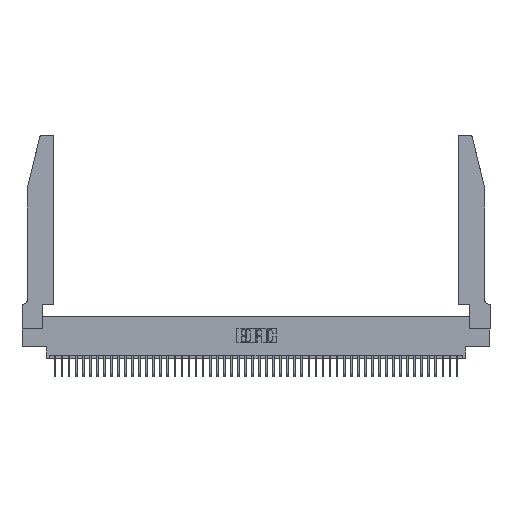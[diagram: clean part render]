
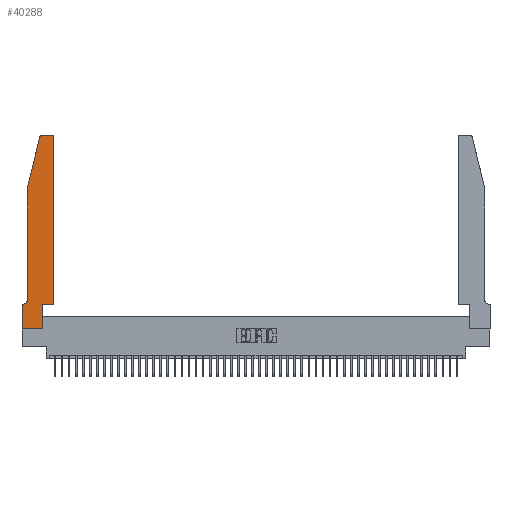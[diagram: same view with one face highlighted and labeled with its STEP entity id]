
A CAD part, top view. The second image highlights one B-rep face of the part: STEP entity #40288.
In plain terms, the highlighted planar face has unit normal (0, 0, 1).
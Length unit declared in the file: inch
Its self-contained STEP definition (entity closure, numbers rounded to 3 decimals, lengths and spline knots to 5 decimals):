
#232 = DIRECTION ( 'NONE',  ( 1., 0., 0. ) ) ;
#491 = DIRECTION ( 'NONE',  ( -1., 0., 0. ) ) ;
#515 = PLANE ( 'NONE',  #5694 ) ;
#577 = ORIENTED_EDGE ( 'NONE', *, *, #37144, .T. ) ;
#1815 = DIRECTION ( 'NONE',  ( 1., 0., 0. ) ) ;
#2448 = ORIENTED_EDGE ( 'NONE', *, *, #42731, .T. ) ;
#2452 = VERTEX_POINT ( 'NONE', #23916 ) ;
#2727 = DIRECTION ( 'NONE',  ( 0., -1., 0. ) ) ;
#2788 = CARTESIAN_POINT ( 'NONE',  ( 0.4505, 0.35, 0.37 ) ) ;
#2880 = ORIENTED_EDGE ( 'NONE', *, *, #31322, .T. ) ;
#3870 = EDGE_CURVE ( 'NONE', #26052, #6404, #36049, .T. ) ;
#3919 = LINE ( 'NONE', #22028, #32597 ) ;
#4111 = DIRECTION ( 'NONE',  ( 0., 0., 1. ) ) ;
#4376 = VERTEX_POINT ( 'NONE', #30611 ) ;
#5043 = VERTEX_POINT ( 'NONE', #2788 ) ;
#5694 = AXIS2_PLACEMENT_3D ( 'NONE', #25688, #4111, #29270 ) ;
#5755 = VECTOR ( 'NONE', #32651, 39.37008 ) ;
#6404 = VERTEX_POINT ( 'NONE', #38678 ) ;
#6987 = ORIENTED_EDGE ( 'NONE', *, *, #38948, .T. ) ;
#7701 = CARTESIAN_POINT ( 'NONE',  ( 0.25487, 2.72718, 0.37 ) ) ;
#8068 = DIRECTION ( 'NONE',  ( 1., 0., 0. ) ) ;
#8474 = VECTOR ( 'NONE', #2727, 39.37008 ) ;
#9667 = EDGE_CURVE ( 'NONE', #31623, #13768, #30006, .T. ) ;
#9889 = CARTESIAN_POINT ( 'NONE',  ( 0.0755, 0.42, 0.37 ) ) ;
#11113 = CARTESIAN_POINT ( 'NONE',  ( 0.2865, 0.35, 0.37 ) ) ;
#11313 = ORIENTED_EDGE ( 'NONE', *, *, #3870, .T. ) ;
#12363 = LINE ( 'NONE', #14494, #39859 ) ;
#13269 = CARTESIAN_POINT ( 'NONE',  ( 0.0055, 0.42, 0.37 ) ) ;
#13534 = VECTOR ( 'NONE', #232, 39.37008 ) ;
#13580 = CARTESIAN_POINT ( 'NONE',  ( 0.4505, 0.35, 0.37 ) ) ;
#13768 = VERTEX_POINT ( 'NONE', #7701 ) ;
#14494 = CARTESIAN_POINT ( 'NONE',  ( 0.2605, 2.75, 0.37 ) ) ;
#15969 = CARTESIAN_POINT ( 'NONE',  ( 0.284, 2.72, 0.37 ) ) ;
#16148 = VERTEX_POINT ( 'NONE', #22478 ) ;
#16163 = LINE ( 'NONE', #13580, #34144 ) ;
#16466 = DIRECTION ( 'NONE',  ( -0.239, -0.971, 0. ) ) ;
#16899 = DIRECTION ( 'NONE',  ( -1., 0., 0. ) ) ;
#17217 = DIRECTION ( 'NONE',  ( 0., 1., 0. ) ) ;
#17283 = ORIENTED_EDGE ( 'NONE', *, *, #19075, .T. ) ;
#17395 = LINE ( 'NONE', #36829, #36491 ) ;
#17997 = CARTESIAN_POINT ( 'NONE',  ( 0.4505, 0.35, 0.37 ) ) ;
#18121 = DIRECTION ( 'NONE',  ( -1., 0., 0. ) ) ;
#18249 = LINE ( 'NONE', #41545, #36187 ) ;
#18891 = ORIENTED_EDGE ( 'NONE', *, *, #32933, .T. ) ;
#19075 = EDGE_CURVE ( 'NONE', #22794, #26052, #3919, .T. ) ;
#19356 = VERTEX_POINT ( 'NONE', #20122 ) ;
#19609 = DIRECTION ( 'NONE',  ( 1., 0., 0. ) ) ;
#20122 = CARTESIAN_POINT ( 'NONE',  ( 0.2865, 0., 0.37 ) ) ;
#20269 = VECTOR ( 'NONE', #16466, 39.37008 ) ;
#22022 = ORIENTED_EDGE ( 'NONE', *, *, #9667, .T. ) ;
#22028 = CARTESIAN_POINT ( 'NONE',  ( 0.0755, 0.35, 0.37 ) ) ;
#22478 = CARTESIAN_POINT ( 'NONE',  ( 0.0755, 2., 0.37 ) ) ;
#22794 = VERTEX_POINT ( 'NONE', #41935 ) ;
#23113 = LINE ( 'NONE', #17997, #13534 ) ;
#23359 = DIRECTION ( 'NONE',  ( 0., 0., 1. ) ) ;
#23916 = CARTESIAN_POINT ( 'NONE',  ( 0.2865, 0.35, 0.37 ) ) ;
#24257 = CARTESIAN_POINT ( 'NONE',  ( 0., 0., 0.37 ) ) ;
#25688 = CARTESIAN_POINT ( 'NONE',  ( 0., 0.35, 0.37 ) ) ;
#26052 = VERTEX_POINT ( 'NONE', #31413 ) ;
#26905 = ORIENTED_EDGE ( 'NONE', *, *, #43058, .T. ) ;
#27730 = EDGE_LOOP ( 'NONE', ( #46224, #22022, #577, #2448, #30096, #17283, #11313, #45237, #26905, #2880, #18891, #6987 ) ) ;
#29270 = DIRECTION ( 'NONE',  ( 1., 0., 0. ) ) ;
#30006 = CIRCLE ( 'NONE', #45775, 0.03 ) ;
#30096 = ORIENTED_EDGE ( 'NONE', *, *, #31067, .T. ) ;
#30611 = CARTESIAN_POINT ( 'NONE',  ( 0.4505, 2.72, 0.37 ) ) ;
#30907 = LINE ( 'NONE', #45097, #20269 ) ;
#31067 = EDGE_CURVE ( 'NONE', #31652, #22794, #33255, .T. ) ;
#31322 = EDGE_CURVE ( 'NONE', #2452, #5043, #23113, .T. ) ;
#31413 = CARTESIAN_POINT ( 'NONE',  ( 0., 0.35, 0.37 ) ) ;
#31623 = VERTEX_POINT ( 'NONE', #41265 ) ;
#31652 = VERTEX_POINT ( 'NONE', #9889 ) ;
#31798 = EDGE_CURVE ( 'NONE', #34210, #31623, #12363, .T. ) ;
#32597 = VECTOR ( 'NONE', #491, 39.37008 ) ;
#32651 = DIRECTION ( 'NONE',  ( 0., 1., 0. ) ) ;
#32933 = EDGE_CURVE ( 'NONE', #5043, #4376, #16163, .T. ) ;
#33255 = CIRCLE ( 'NONE', #46022, 0.07 ) ;
#34144 = VECTOR ( 'NONE', #17217, 39.37008 ) ;
#34210 = VERTEX_POINT ( 'NONE', #41408 ) ;
#34217 = FACE_OUTER_BOUND ( 'NONE', #27730, .T. ) ;
#36049 = LINE ( 'NONE', #24257, #8474 ) ;
#36187 = VECTOR ( 'NONE', #45154, 39.37008 ) ;
#36491 = VECTOR ( 'NONE', #8068, 39.37008 ) ;
#36829 = CARTESIAN_POINT ( 'NONE',  ( 0., 0., 0.37 ) ) ;
#37144 = EDGE_CURVE ( 'NONE', #13768, #16148, #30907, .T. ) ;
#38356 = DIRECTION ( 'NONE',  ( 0., 0., -1. ) ) ;
#38678 = CARTESIAN_POINT ( 'NONE',  ( 0., 0., 0.37 ) ) ;
#38948 = EDGE_CURVE ( 'NONE', #4376, #34210, #40919, .T. ) ;
#39768 = EDGE_CURVE ( 'NONE', #6404, #19356, #17395, .T. ) ;
#39859 = VECTOR ( 'NONE', #18121, 39.37008 ) ;
#40288 = ADVANCED_FACE ( 'NONE', ( #34217 ), #515, .T. ) ;
#40919 = CIRCLE ( 'NONE', #46254, 0.03 ) ;
#40995 = DIRECTION ( 'NONE',  ( 0., 0., 1. ) ) ;
#41265 = CARTESIAN_POINT ( 'NONE',  ( 0.284, 2.75, 0.37 ) ) ;
#41408 = CARTESIAN_POINT ( 'NONE',  ( 0.4205, 2.75, 0.37 ) ) ;
#41545 = CARTESIAN_POINT ( 'NONE',  ( 0.0755, 2., 0.37 ) ) ;
#41935 = CARTESIAN_POINT ( 'NONE',  ( 0.0055, 0.35, 0.37 ) ) ;
#42731 = EDGE_CURVE ( 'NONE', #16148, #31652, #18249, .T. ) ;
#43058 = EDGE_CURVE ( 'NONE', #19356, #2452, #43954, .T. ) ;
#43954 = LINE ( 'NONE', #11113, #5755 ) ;
#44782 = CARTESIAN_POINT ( 'NONE',  ( 0.4205, 2.72, 0.37 ) ) ;
#45097 = CARTESIAN_POINT ( 'NONE',  ( 0.0755, 2., 0.37 ) ) ;
#45154 = DIRECTION ( 'NONE',  ( 0., -1., 0. ) ) ;
#45237 = ORIENTED_EDGE ( 'NONE', *, *, #39768, .T. ) ;
#45775 = AXIS2_PLACEMENT_3D ( 'NONE', #15969, #40995, #19609 ) ;
#46022 = AXIS2_PLACEMENT_3D ( 'NONE', #13269, #38356, #16899 ) ;
#46224 = ORIENTED_EDGE ( 'NONE', *, *, #31798, .T. ) ;
#46254 = AXIS2_PLACEMENT_3D ( 'NONE', #44782, #23359, #1815 ) ;
